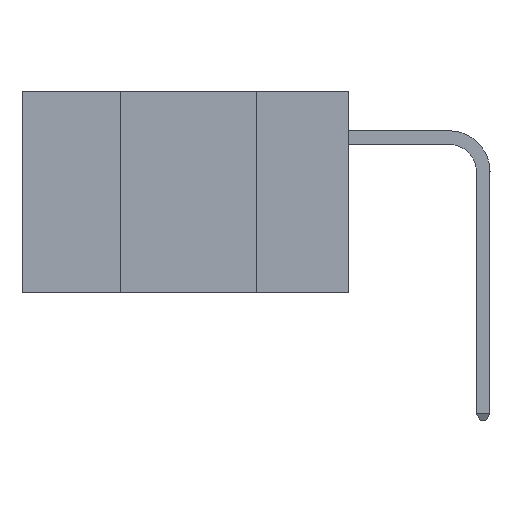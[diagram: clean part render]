
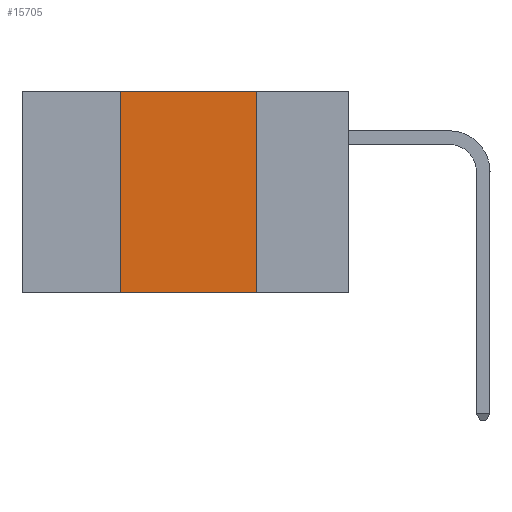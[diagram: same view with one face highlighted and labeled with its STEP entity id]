
A CAD part, left-side view. The second image highlights one B-rep face of the part: STEP entity #15705.
In plain terms, the highlighted planar face has unit normal (-1, 0, 0).
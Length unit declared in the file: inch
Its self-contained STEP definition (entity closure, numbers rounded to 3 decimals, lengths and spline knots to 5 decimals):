
#134 = DIRECTION ( 'NONE',  ( 0., 0., 1. ) ) ;
#322 = ORIENTED_EDGE ( 'NONE', *, *, #8490, .F. ) ;
#689 = AXIS2_PLACEMENT_3D ( 'NONE', #16092, #17433, #9443 ) ;
#1197 = VERTEX_POINT ( 'NONE', #16424 ) ;
#2131 = LINE ( 'NONE', #14697, #12963 ) ;
#2221 = CARTESIAN_POINT ( 'NONE',  ( 0., 0.17, 0. ) ) ;
#2880 = VERTEX_POINT ( 'NONE', #14912 ) ;
#2914 = CARTESIAN_POINT ( 'NONE',  ( 0., 0.42, 0. ) ) ;
#4895 = CARTESIAN_POINT ( 'NONE',  ( 0., 0.6, -0.37 ) ) ;
#5037 = LINE ( 'NONE', #4895, #15391 ) ;
#5298 = VERTEX_POINT ( 'NONE', #14287 ) ;
#5852 = DIRECTION ( 'NONE',  ( 0., 0., -1. ) ) ;
#5956 = VECTOR ( 'NONE', #5852, 39.37008 ) ;
#7862 = LINE ( 'NONE', #2914, #14593 ) ;
#7976 = PLANE ( 'NONE',  #689 ) ;
#7986 = DIRECTION ( 'NONE',  ( 0., -1., 0. ) ) ;
#8490 = EDGE_CURVE ( 'NONE', #12975, #2880, #13139, .T. ) ;
#9443 = DIRECTION ( 'NONE',  ( 0., 0., -1. ) ) ;
#11214 = EDGE_CURVE ( 'NONE', #5298, #1197, #7862, .T. ) ;
#11395 = ORIENTED_EDGE ( 'NONE', *, *, #13579, .T. ) ;
#11737 = DIRECTION ( 'NONE',  ( 0., -1., 0. ) ) ;
#12963 = VECTOR ( 'NONE', #7986, 39.37008 ) ;
#12975 = VERTEX_POINT ( 'NONE', #2221 ) ;
#13139 = LINE ( 'NONE', #15295, #5956 ) ;
#13579 = EDGE_CURVE ( 'NONE', #5298, #2880, #5037, .T. ) ;
#13841 = EDGE_LOOP ( 'NONE', ( #322, #16776, #17284, #11395 ) ) ;
#14287 = CARTESIAN_POINT ( 'NONE',  ( 0., 0.42, -0.37 ) ) ;
#14456 = FACE_OUTER_BOUND ( 'NONE', #13841, .T. ) ;
#14593 = VECTOR ( 'NONE', #134, 39.37008 ) ;
#14697 = CARTESIAN_POINT ( 'NONE',  ( 0., 0.6, 0. ) ) ;
#14912 = CARTESIAN_POINT ( 'NONE',  ( 0., 0.17, -0.37 ) ) ;
#15295 = CARTESIAN_POINT ( 'NONE',  ( 0., 0.17, 0. ) ) ;
#15391 = VECTOR ( 'NONE', #11737, 39.37008 ) ;
#15705 = ADVANCED_FACE ( 'NONE', ( #14456 ), #7976, .F. ) ;
#16092 = CARTESIAN_POINT ( 'NONE',  ( 0., 0.6, 0. ) ) ;
#16424 = CARTESIAN_POINT ( 'NONE',  ( 0., 0.42, 0. ) ) ;
#16776 = ORIENTED_EDGE ( 'NONE', *, *, #17011, .F. ) ;
#17011 = EDGE_CURVE ( 'NONE', #1197, #12975, #2131, .T. ) ;
#17284 = ORIENTED_EDGE ( 'NONE', *, *, #11214, .F. ) ;
#17433 = DIRECTION ( 'NONE',  ( 1., 0., 0. ) ) ;
